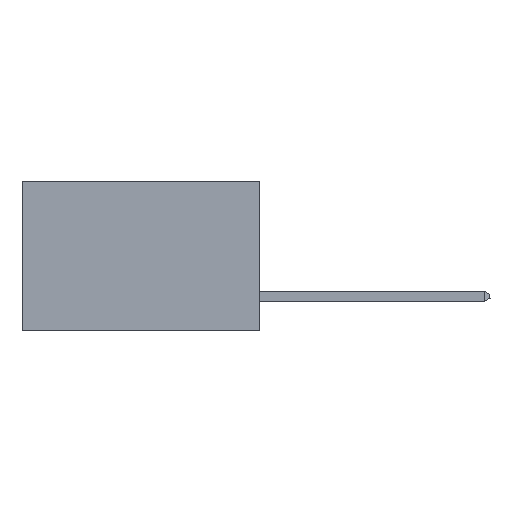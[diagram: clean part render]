
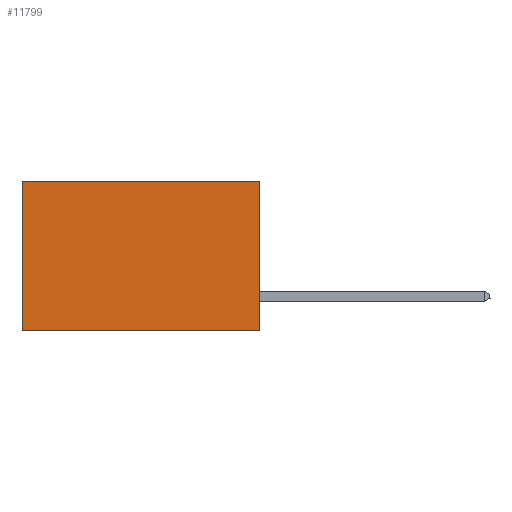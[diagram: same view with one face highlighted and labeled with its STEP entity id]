
A CAD part, left-side view. The second image highlights one B-rep face of the part: STEP entity #11799.
In plain terms, the highlighted planar face has unit normal (-1, 0, 0).
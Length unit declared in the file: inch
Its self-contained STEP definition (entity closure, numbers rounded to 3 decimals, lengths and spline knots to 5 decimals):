
#359 = VERTEX_POINT ( 'NONE', #6493 ) ;
#417 = DIRECTION ( 'NONE',  ( 0., 1., 0. ) ) ;
#733 = VERTEX_POINT ( 'NONE', #16194 ) ;
#1423 = CARTESIAN_POINT ( 'NONE',  ( 0.277, 0., -0.37 ) ) ;
#1768 = PLANE ( 'NONE',  #3232 ) ;
#1971 = VECTOR ( 'NONE', #16774, 39.37008 ) ;
#3232 = AXIS2_PLACEMENT_3D ( 'NONE', #17500, #11922, #3249 ) ;
#3249 = DIRECTION ( 'NONE',  ( 0., 0., -1. ) ) ;
#3787 = FACE_OUTER_BOUND ( 'NONE', #10314, .T. ) ;
#4202 = VECTOR ( 'NONE', #16319, 39.37008 ) ;
#4419 = CARTESIAN_POINT ( 'NONE',  ( 0.277, 0., -0.37 ) ) ;
#5798 = ORIENTED_EDGE ( 'NONE', *, *, #6686, .T. ) ;
#6254 = ORIENTED_EDGE ( 'NONE', *, *, #13083, .F. ) ;
#6493 = CARTESIAN_POINT ( 'NONE',  ( 0.277, 0.59, -0.37 ) ) ;
#6686 = EDGE_CURVE ( 'NONE', #7575, #359, #13491, .T. ) ;
#7575 = VERTEX_POINT ( 'NONE', #16242 ) ;
#10314 = EDGE_LOOP ( 'NONE', ( #5798, #6254, #10546, #10963 ) ) ;
#10546 = ORIENTED_EDGE ( 'NONE', *, *, #18430, .F. ) ;
#10659 = CARTESIAN_POINT ( 'NONE',  ( 0.277, 0., 0. ) ) ;
#10963 = ORIENTED_EDGE ( 'NONE', *, *, #17344, .T. ) ;
#11799 = ADVANCED_FACE ( 'NONE', ( #3787 ), #1768, .F. ) ;
#11922 = DIRECTION ( 'NONE',  ( 1., 0., 0. ) ) ;
#12008 = VECTOR ( 'NONE', #14465, 39.37008 ) ;
#12237 = VERTEX_POINT ( 'NONE', #1423 ) ;
#12875 = LINE ( 'NONE', #4419, #12008 ) ;
#13083 = EDGE_CURVE ( 'NONE', #12237, #359, #14701, .T. ) ;
#13491 = LINE ( 'NONE', #17363, #1971 ) ;
#14465 = DIRECTION ( 'NONE',  ( 0., 0., -1. ) ) ;
#14701 = LINE ( 'NONE', #14898, #4202 ) ;
#14898 = CARTESIAN_POINT ( 'NONE',  ( 0.277, 0., -0.37 ) ) ;
#16194 = CARTESIAN_POINT ( 'NONE',  ( 0.277, 0., 0. ) ) ;
#16242 = CARTESIAN_POINT ( 'NONE',  ( 0.277, 0.59, 0. ) ) ;
#16319 = DIRECTION ( 'NONE',  ( 0., 1., 0. ) ) ;
#16774 = DIRECTION ( 'NONE',  ( 0., 0., -1. ) ) ;
#16898 = VECTOR ( 'NONE', #417, 39.37008 ) ;
#17317 = LINE ( 'NONE', #10659, #16898 ) ;
#17344 = EDGE_CURVE ( 'NONE', #733, #7575, #17317, .T. ) ;
#17363 = CARTESIAN_POINT ( 'NONE',  ( 0.277, 0.59, -0.37 ) ) ;
#17500 = CARTESIAN_POINT ( 'NONE',  ( 0.277, 0., -0.37 ) ) ;
#18430 = EDGE_CURVE ( 'NONE', #733, #12237, #12875, .T. ) ;
